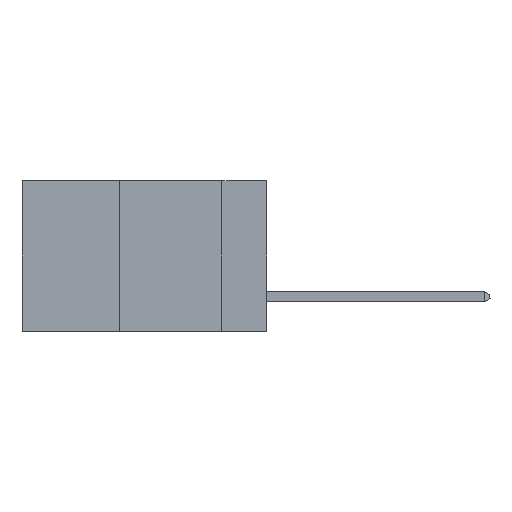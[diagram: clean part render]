
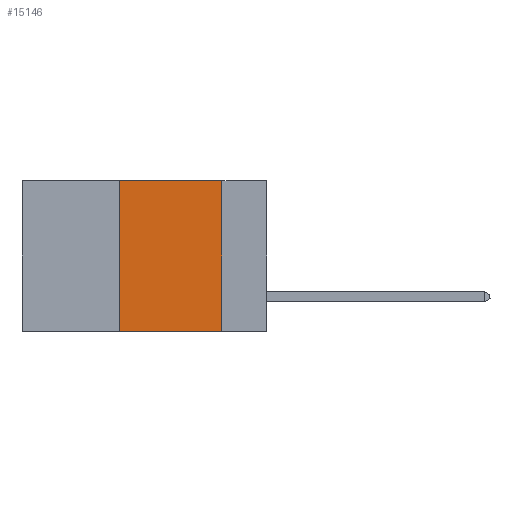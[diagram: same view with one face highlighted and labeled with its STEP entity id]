
A CAD part, left-side view. The second image highlights one B-rep face of the part: STEP entity #15146.
In plain terms, the highlighted planar face has unit normal (-1, 0, 0).
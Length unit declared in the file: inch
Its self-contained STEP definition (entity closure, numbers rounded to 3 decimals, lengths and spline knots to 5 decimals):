
#2016 = FACE_OUTER_BOUND ( 'NONE', #47055, .T. ) ;
#6128 = DIRECTION ( 'NONE',  ( 0., 0., -1. ) ) ;
#7093 = VERTEX_POINT ( 'NONE', #45460 ) ;
#7428 = EDGE_CURVE ( 'NONE', #7093, #10723, #49650, .T. ) ;
#7690 = ORIENTED_EDGE ( 'NONE', *, *, #7428, .T. ) ;
#10581 = CARTESIAN_POINT ( 'NONE',  ( 0., 0.11, -0.37 ) ) ;
#10723 = VERTEX_POINT ( 'NONE', #10581 ) ;
#11127 = DIRECTION ( 'NONE',  ( 0., -1., 0. ) ) ;
#12454 = VECTOR ( 'NONE', #6128, 39.37008 ) ;
#14916 = LINE ( 'NONE', #44537, #12454 ) ;
#15146 = ADVANCED_FACE ( 'NONE', ( #2016 ), #44044, .F. ) ;
#15323 = DIRECTION ( 'NONE',  ( 0., 0., 1. ) ) ;
#15457 = CARTESIAN_POINT ( 'NONE',  ( 0., 0.6, -0.37 ) ) ;
#17708 = CARTESIAN_POINT ( 'NONE',  ( 0., 0.36, 0. ) ) ;
#17938 = CARTESIAN_POINT ( 'NONE',  ( 0., 0.11, 0. ) ) ;
#19661 = AXIS2_PLACEMENT_3D ( 'NONE', #24912, #40350, #32956 ) ;
#24912 = CARTESIAN_POINT ( 'NONE',  ( 0., 0.6, 0. ) ) ;
#27368 = EDGE_CURVE ( 'NONE', #41768, #10723, #14916, .T. ) ;
#30639 = EDGE_CURVE ( 'NONE', #44859, #41768, #39741, .T. ) ;
#32395 = ORIENTED_EDGE ( 'NONE', *, *, #42561, .F. ) ;
#32956 = DIRECTION ( 'NONE',  ( 0., 0., -1. ) ) ;
#34274 = CARTESIAN_POINT ( 'NONE',  ( 0., 0.36, 0. ) ) ;
#39741 = LINE ( 'NONE', #45158, #46348 ) ;
#40350 = DIRECTION ( 'NONE',  ( 1., 0., 0. ) ) ;
#41249 = VECTOR ( 'NONE', #15323, 39.37008 ) ;
#41768 = VERTEX_POINT ( 'NONE', #17938 ) ;
#41954 = DIRECTION ( 'NONE',  ( 0., -1., 0. ) ) ;
#42561 = EDGE_CURVE ( 'NONE', #7093, #44859, #47290, .T. ) ;
#42725 = ORIENTED_EDGE ( 'NONE', *, *, #27368, .F. ) ;
#43576 = VECTOR ( 'NONE', #41954, 39.37008 ) ;
#44044 = PLANE ( 'NONE',  #19661 ) ;
#44537 = CARTESIAN_POINT ( 'NONE',  ( 0., 0.11, 0. ) ) ;
#44859 = VERTEX_POINT ( 'NONE', #17708 ) ;
#45158 = CARTESIAN_POINT ( 'NONE',  ( 0., 0.6, 0. ) ) ;
#45460 = CARTESIAN_POINT ( 'NONE',  ( 0., 0.36, -0.37 ) ) ;
#46348 = VECTOR ( 'NONE', #11127, 39.37008 ) ;
#47055 = EDGE_LOOP ( 'NONE', ( #42725, #48857, #32395, #7690 ) ) ;
#47290 = LINE ( 'NONE', #34274, #41249 ) ;
#48857 = ORIENTED_EDGE ( 'NONE', *, *, #30639, .F. ) ;
#49650 = LINE ( 'NONE', #15457, #43576 ) ;
